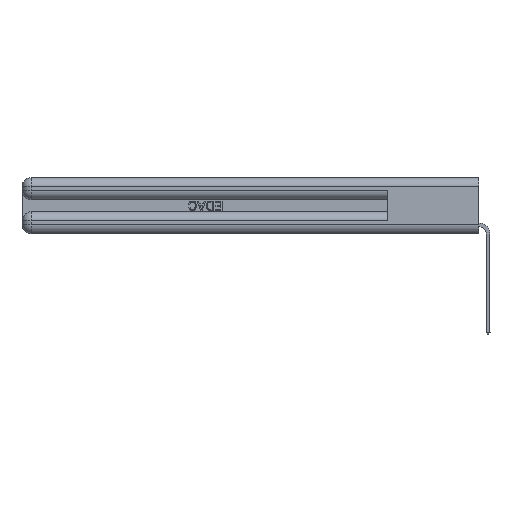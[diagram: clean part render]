
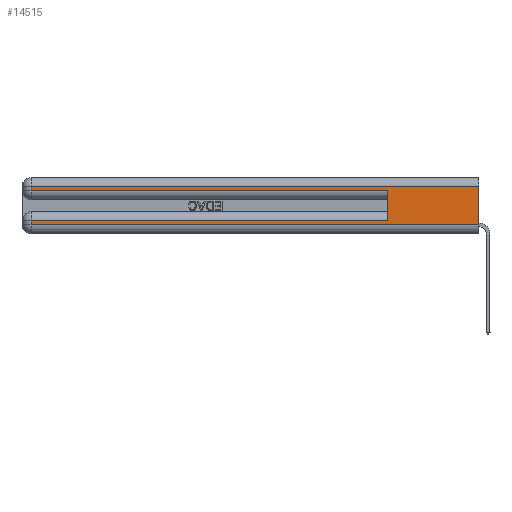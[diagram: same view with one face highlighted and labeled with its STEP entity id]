
A CAD part, left-side view. The second image highlights one B-rep face of the part: STEP entity #14515.
In plain terms, the highlighted planar face has unit normal (-1, 0, 0).
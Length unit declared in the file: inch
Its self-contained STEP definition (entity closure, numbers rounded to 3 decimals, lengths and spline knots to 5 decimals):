
#30 = VECTOR ( 'NONE', #21953, 39.37008 ) ;
#106 = CARTESIAN_POINT ( 'NONE',  ( 0., 0., 0.31 ) ) ;
#1444 = VECTOR ( 'NONE', #13937, 39.37008 ) ;
#1501 = VERTEX_POINT ( 'NONE', #106 ) ;
#1880 = EDGE_CURVE ( 'NONE', #3724, #25263, #23491, .T. ) ;
#3048 = VERTEX_POINT ( 'NONE', #11493 ) ;
#3401 = VECTOR ( 'NONE', #27046, 39.37008 ) ;
#3724 = VERTEX_POINT ( 'NONE', #22629 ) ;
#4417 = VECTOR ( 'NONE', #15810, 39.37008 ) ;
#4836 = LINE ( 'NONE', #9038, #3401 ) ;
#4862 = VERTEX_POINT ( 'NONE', #23257 ) ;
#5264 = DIRECTION ( 'NONE',  ( 0., 0., -1. ) ) ;
#5714 = CARTESIAN_POINT ( 'NONE',  ( 0., 2.94, 0.31 ) ) ;
#5972 = ORIENTED_EDGE ( 'NONE', *, *, #26574, .F. ) ;
#6248 = CARTESIAN_POINT ( 'NONE',  ( 0., 0., 0.06 ) ) ;
#7076 = FACE_OUTER_BOUND ( 'NONE', #22479, .T. ) ;
#7482 = LINE ( 'NONE', #26399, #13575 ) ;
#7595 = LINE ( 'NONE', #11636, #1444 ) ;
#8185 = ORIENTED_EDGE ( 'NONE', *, *, #11958, .T. ) ;
#9038 = CARTESIAN_POINT ( 'NONE',  ( 0., 0., 0.31 ) ) ;
#9372 = VERTEX_POINT ( 'NONE', #5714 ) ;
#9782 = CARTESIAN_POINT ( 'NONE',  ( 0., 0., 0.37 ) ) ;
#10644 = EDGE_CURVE ( 'NONE', #9372, #4862, #22486, .T. ) ;
#11493 = CARTESIAN_POINT ( 'NONE',  ( 0., 2.94, 0.06 ) ) ;
#11636 = CARTESIAN_POINT ( 'NONE',  ( 0., 0., 0.06 ) ) ;
#11958 = EDGE_CURVE ( 'NONE', #3048, #25253, #7595, .T. ) ;
#12069 = DIRECTION ( 'NONE',  ( 0., 0., -1. ) ) ;
#12925 = VECTOR ( 'NONE', #13548, 39.37008 ) ;
#12958 = DIRECTION ( 'NONE',  ( 0., 0., 1. ) ) ;
#13548 = DIRECTION ( 'NONE',  ( 0., -1., 0. ) ) ;
#13575 = VECTOR ( 'NONE', #12958, 39.37008 ) ;
#13669 = ORIENTED_EDGE ( 'NONE', *, *, #28948, .T. ) ;
#13937 = DIRECTION ( 'NONE',  ( 0., -1., 0. ) ) ;
#14356 = ORIENTED_EDGE ( 'NONE', *, *, #15577, .T. ) ;
#14515 = ADVANCED_FACE ( 'NONE', ( #7076 ), #21004, .F. ) ;
#15295 = VERTEX_POINT ( 'NONE', #19318 ) ;
#15461 = CARTESIAN_POINT ( 'NONE',  ( 0., 2.94, 0.085 ) ) ;
#15577 = EDGE_CURVE ( 'NONE', #1501, #9372, #4836, .T. ) ;
#15735 = LINE ( 'NONE', #16657, #26929 ) ;
#15810 = DIRECTION ( 'NONE',  ( 0., 0., -1. ) ) ;
#15962 = ORIENTED_EDGE ( 'NONE', *, *, #21306, .T. ) ;
#16657 = CARTESIAN_POINT ( 'NONE',  ( 0., 0., 0.37 ) ) ;
#17300 = VECTOR ( 'NONE', #22766, 39.37008 ) ;
#18550 = ORIENTED_EDGE ( 'NONE', *, *, #27106, .F. ) ;
#19318 = CARTESIAN_POINT ( 'NONE',  ( 0., 0.6, 0.285 ) ) ;
#21004 = PLANE ( 'NONE',  #26618 ) ;
#21306 = EDGE_CURVE ( 'NONE', #25263, #3048, #22478, .T. ) ;
#21953 = DIRECTION ( 'NONE',  ( 0., 1., 0. ) ) ;
#22478 = LINE ( 'NONE', #26949, #4417 ) ;
#22479 = EDGE_LOOP ( 'NONE', ( #5972, #14356, #24227, #13669, #18550, #27446, #15962, #8185 ) ) ;
#22486 = LINE ( 'NONE', #25056, #17300 ) ;
#22629 = CARTESIAN_POINT ( 'NONE',  ( 0., 0.6, 0.085 ) ) ;
#22766 = DIRECTION ( 'NONE',  ( 0., 0., -1. ) ) ;
#23257 = CARTESIAN_POINT ( 'NONE',  ( 0., 2.94, 0.285 ) ) ;
#23491 = LINE ( 'NONE', #26506, #30 ) ;
#24227 = ORIENTED_EDGE ( 'NONE', *, *, #10644, .T. ) ;
#24839 = LINE ( 'NONE', #29232, #12925 ) ;
#25056 = CARTESIAN_POINT ( 'NONE',  ( 0., 2.94, 0.37 ) ) ;
#25253 = VERTEX_POINT ( 'NONE', #6248 ) ;
#25263 = VERTEX_POINT ( 'NONE', #15461 ) ;
#25512 = DIRECTION ( 'NONE',  ( 1., 0., 0. ) ) ;
#26399 = CARTESIAN_POINT ( 'NONE',  ( 0., 0.6, 0.145 ) ) ;
#26506 = CARTESIAN_POINT ( 'NONE',  ( 0., 0., 0.085 ) ) ;
#26574 = EDGE_CURVE ( 'NONE', #1501, #25253, #15735, .T. ) ;
#26618 = AXIS2_PLACEMENT_3D ( 'NONE', #9782, #25512, #12069 ) ;
#26929 = VECTOR ( 'NONE', #5264, 39.37008 ) ;
#26949 = CARTESIAN_POINT ( 'NONE',  ( 0., 2.94, 0.37 ) ) ;
#27046 = DIRECTION ( 'NONE',  ( 0., 1., 0. ) ) ;
#27106 = EDGE_CURVE ( 'NONE', #3724, #15295, #7482, .T. ) ;
#27446 = ORIENTED_EDGE ( 'NONE', *, *, #1880, .T. ) ;
#28948 = EDGE_CURVE ( 'NONE', #4862, #15295, #24839, .T. ) ;
#29232 = CARTESIAN_POINT ( 'NONE',  ( 0., 0., 0.285 ) ) ;
